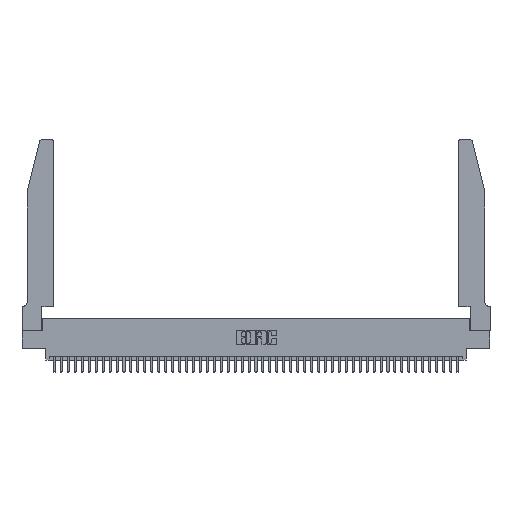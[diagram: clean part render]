
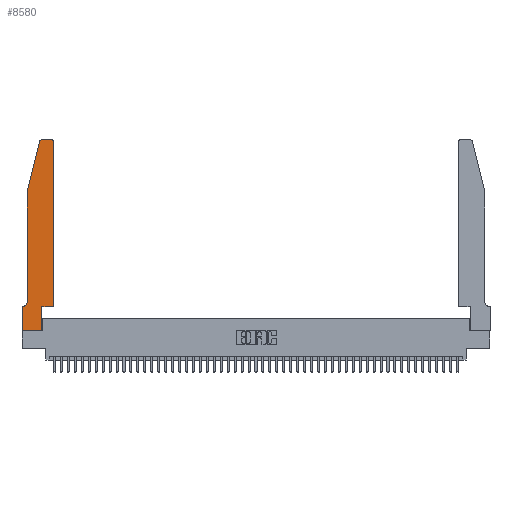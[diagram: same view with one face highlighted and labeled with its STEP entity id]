
A CAD part, top view. The second image highlights one B-rep face of the part: STEP entity #8580.
In plain terms, the highlighted planar face has unit normal (0, 0, 1).
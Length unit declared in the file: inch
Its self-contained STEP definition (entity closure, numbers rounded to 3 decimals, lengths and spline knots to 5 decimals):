
#132 = VERTEX_POINT ( 'NONE', #42486 ) ;
#834 = CIRCLE ( 'NONE', #31912, 0.03 ) ;
#1106 = CARTESIAN_POINT ( 'NONE',  ( 0., 0., 0.37 ) ) ;
#2917 = VERTEX_POINT ( 'NONE', #35390 ) ;
#2929 = CARTESIAN_POINT ( 'NONE',  ( 0.4205, 2.72, 0.37 ) ) ;
#3760 = VERTEX_POINT ( 'NONE', #21811 ) ;
#4550 = ORIENTED_EDGE ( 'NONE', *, *, #22348, .T. ) ;
#4693 = CARTESIAN_POINT ( 'NONE',  ( 0.0055, 0.42, 0.37 ) ) ;
#5266 = VERTEX_POINT ( 'NONE', #18754 ) ;
#5295 = LINE ( 'NONE', #35172, #44310 ) ;
#5703 = VECTOR ( 'NONE', #44625, 39.37008 ) ;
#5839 = EDGE_CURVE ( 'NONE', #15557, #23111, #25914, .T. ) ;
#6757 = DIRECTION ( 'NONE',  ( 1., 0., 0. ) ) ;
#6848 = ORIENTED_EDGE ( 'NONE', *, *, #29968, .T. ) ;
#7638 = ORIENTED_EDGE ( 'NONE', *, *, #12763, .T. ) ;
#7735 = EDGE_CURVE ( 'NONE', #25739, #42822, #35230, .T. ) ;
#8537 = DIRECTION ( 'NONE',  ( -1., 0., 0. ) ) ;
#8580 = ADVANCED_FACE ( 'NONE', ( #16237 ), #31673, .T. ) ;
#8931 = CARTESIAN_POINT ( 'NONE',  ( 0.4505, 2.72, 0.37 ) ) ;
#8952 = LINE ( 'NONE', #37262, #20262 ) ;
#9004 = CARTESIAN_POINT ( 'NONE',  ( 0., 0.35, 0.37 ) ) ;
#12284 = LINE ( 'NONE', #43491, #41237 ) ;
#12763 = EDGE_CURVE ( 'NONE', #23111, #25739, #44737, .T. ) ;
#12833 = DIRECTION ( 'NONE',  ( 1., 0., 0. ) ) ;
#12917 = ORIENTED_EDGE ( 'NONE', *, *, #25818, .T. ) ;
#15086 = CARTESIAN_POINT ( 'NONE',  ( 0.4505, 0.35, 0.37 ) ) ;
#15441 = CARTESIAN_POINT ( 'NONE',  ( 0.2865, 0.35, 0.37 ) ) ;
#15557 = VERTEX_POINT ( 'NONE', #46630 ) ;
#15798 = ORIENTED_EDGE ( 'NONE', *, *, #5839, .T. ) ;
#16198 = ORIENTED_EDGE ( 'NONE', *, *, #20992, .T. ) ;
#16237 = FACE_OUTER_BOUND ( 'NONE', #33613, .T. ) ;
#16863 = EDGE_CURVE ( 'NONE', #2917, #25178, #27881, .T. ) ;
#18754 = CARTESIAN_POINT ( 'NONE',  ( 0.284, 2.75, 0.37 ) ) ;
#18913 = LINE ( 'NONE', #26520, #27789 ) ;
#18953 = DIRECTION ( 'NONE',  ( -1., 0., 0. ) ) ;
#20262 = VECTOR ( 'NONE', #41040, 39.37008 ) ;
#20304 = ORIENTED_EDGE ( 'NONE', *, *, #16863, .T. ) ;
#20992 = EDGE_CURVE ( 'NONE', #42822, #34076, #37755, .T. ) ;
#21811 = CARTESIAN_POINT ( 'NONE',  ( 0.0055, 0.35, 0.37 ) ) ;
#22071 = CARTESIAN_POINT ( 'NONE',  ( 0.4505, 0.35, 0.37 ) ) ;
#22348 = EDGE_CURVE ( 'NONE', #5266, #48985, #834, .T. ) ;
#22619 = CARTESIAN_POINT ( 'NONE',  ( 0.284, 2.72, 0.37 ) ) ;
#23111 = VERTEX_POINT ( 'NONE', #15441 ) ;
#23603 = AXIS2_PLACEMENT_3D ( 'NONE', #9004, #35458, #12833 ) ;
#23971 = DIRECTION ( 'NONE',  ( 0., -1., 0. ) ) ;
#24577 = EDGE_CURVE ( 'NONE', #25178, #15557, #12284, .T. ) ;
#24714 = VECTOR ( 'NONE', #25782, 39.37008 ) ;
#24727 = DIRECTION ( 'NONE',  ( 1., 0., 0. ) ) ;
#25178 = VERTEX_POINT ( 'NONE', #33298 ) ;
#25739 = VERTEX_POINT ( 'NONE', #32753 ) ;
#25782 = DIRECTION ( 'NONE',  ( 0., 1., 0. ) ) ;
#25818 = EDGE_CURVE ( 'NONE', #48985, #132, #34665, .T. ) ;
#25914 = LINE ( 'NONE', #29576, #24714 ) ;
#26397 = VECTOR ( 'NONE', #37670, 39.37008 ) ;
#26422 = DIRECTION ( 'NONE',  ( 1., 0., 0. ) ) ;
#26520 = CARTESIAN_POINT ( 'NONE',  ( 0.2605, 2.75, 0.37 ) ) ;
#27789 = VECTOR ( 'NONE', #18953, 39.37008 ) ;
#27881 = LINE ( 'NONE', #1106, #36678 ) ;
#28866 = CIRCLE ( 'NONE', #38839, 0.07 ) ;
#29030 = ORIENTED_EDGE ( 'NONE', *, *, #36569, .T. ) ;
#29470 = DIRECTION ( 'NONE',  ( 0., 0., 1. ) ) ;
#29576 = CARTESIAN_POINT ( 'NONE',  ( 0.2865, 0.35, 0.37 ) ) ;
#29968 = EDGE_CURVE ( 'NONE', #34076, #5266, #18913, .T. ) ;
#30763 = EDGE_CURVE ( 'NONE', #132, #31756, #5295, .T. ) ;
#31206 = DIRECTION ( 'NONE',  ( 0., 0., -1. ) ) ;
#31673 = PLANE ( 'NONE',  #23603 ) ;
#31756 = VERTEX_POINT ( 'NONE', #44650 ) ;
#31912 = AXIS2_PLACEMENT_3D ( 'NONE', #22619, #48960, #26422 ) ;
#32753 = CARTESIAN_POINT ( 'NONE',  ( 0.4505, 0.35, 0.37 ) ) ;
#33075 = CARTESIAN_POINT ( 'NONE',  ( 0.0755, 2., 0.37 ) ) ;
#33179 = EDGE_CURVE ( 'NONE', #31756, #3760, #28866, .T. ) ;
#33298 = CARTESIAN_POINT ( 'NONE',  ( 0., 0., 0.37 ) ) ;
#33357 = CARTESIAN_POINT ( 'NONE',  ( 0.4205, 2.75, 0.37 ) ) ;
#33613 = EDGE_LOOP ( 'NONE', ( #6848, #4550, #12917, #39935, #40675, #29030, #20304, #35757, #15798, #7638, #41492, #16198 ) ) ;
#34076 = VERTEX_POINT ( 'NONE', #33357 ) ;
#34665 = LINE ( 'NONE', #33075, #43496 ) ;
#35172 = CARTESIAN_POINT ( 'NONE',  ( 0.0755, 2., 0.37 ) ) ;
#35230 = LINE ( 'NONE', #15086, #26397 ) ;
#35390 = CARTESIAN_POINT ( 'NONE',  ( 0., 0.35, 0.37 ) ) ;
#35458 = DIRECTION ( 'NONE',  ( 0., 0., 1. ) ) ;
#35669 = AXIS2_PLACEMENT_3D ( 'NONE', #2929, #29470, #6757 ) ;
#35757 = ORIENTED_EDGE ( 'NONE', *, *, #24577, .T. ) ;
#35934 = CARTESIAN_POINT ( 'NONE',  ( 0.25487, 2.72718, 0.37 ) ) ;
#36569 = EDGE_CURVE ( 'NONE', #3760, #2917, #8952, .T. ) ;
#36678 = VECTOR ( 'NONE', #46445, 39.37008 ) ;
#36870 = DIRECTION ( 'NONE',  ( -0.239, -0.971, 0. ) ) ;
#37262 = CARTESIAN_POINT ( 'NONE',  ( 0.0755, 0.35, 0.37 ) ) ;
#37670 = DIRECTION ( 'NONE',  ( 0., 1., 0. ) ) ;
#37755 = CIRCLE ( 'NONE', #35669, 0.03 ) ;
#38839 = AXIS2_PLACEMENT_3D ( 'NONE', #4693, #31206, #8537 ) ;
#39935 = ORIENTED_EDGE ( 'NONE', *, *, #30763, .T. ) ;
#40675 = ORIENTED_EDGE ( 'NONE', *, *, #33179, .T. ) ;
#41040 = DIRECTION ( 'NONE',  ( -1., 0., 0. ) ) ;
#41237 = VECTOR ( 'NONE', #24727, 39.37008 ) ;
#41492 = ORIENTED_EDGE ( 'NONE', *, *, #7735, .T. ) ;
#42486 = CARTESIAN_POINT ( 'NONE',  ( 0.0755, 2., 0.37 ) ) ;
#42822 = VERTEX_POINT ( 'NONE', #8931 ) ;
#43491 = CARTESIAN_POINT ( 'NONE',  ( 0., 0., 0.37 ) ) ;
#43496 = VECTOR ( 'NONE', #36870, 39.37008 ) ;
#44310 = VECTOR ( 'NONE', #23971, 39.37008 ) ;
#44625 = DIRECTION ( 'NONE',  ( 1., 0., 0. ) ) ;
#44650 = CARTESIAN_POINT ( 'NONE',  ( 0.0755, 0.42, 0.37 ) ) ;
#44737 = LINE ( 'NONE', #22071, #5703 ) ;
#46445 = DIRECTION ( 'NONE',  ( 0., -1., 0. ) ) ;
#46630 = CARTESIAN_POINT ( 'NONE',  ( 0.2865, 0., 0.37 ) ) ;
#48960 = DIRECTION ( 'NONE',  ( 0., 0., 1. ) ) ;
#48985 = VERTEX_POINT ( 'NONE', #35934 ) ;
